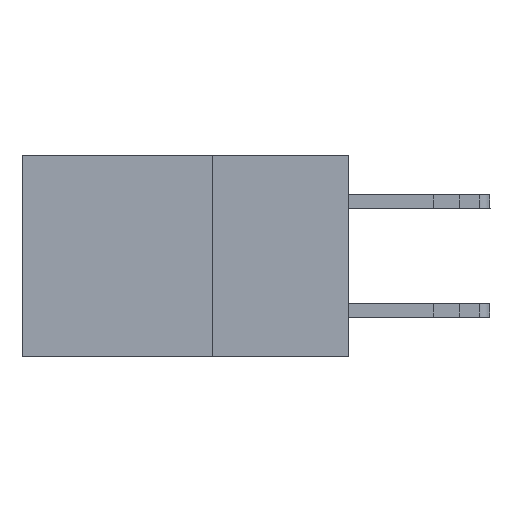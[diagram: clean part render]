
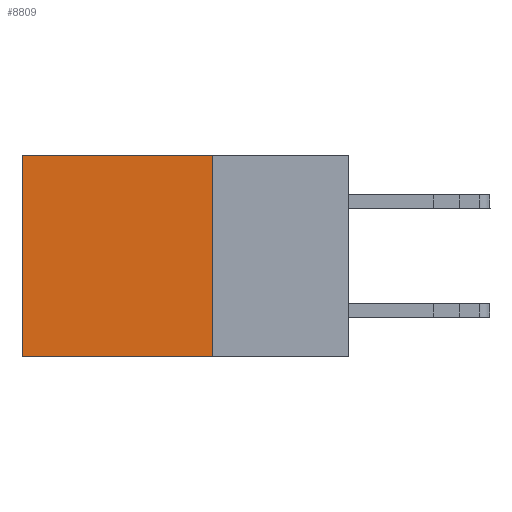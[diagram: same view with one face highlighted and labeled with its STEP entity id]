
A CAD part, left-side view. The second image highlights one B-rep face of the part: STEP entity #8809.
In plain terms, the highlighted planar face has unit normal (-1, 0, 0).
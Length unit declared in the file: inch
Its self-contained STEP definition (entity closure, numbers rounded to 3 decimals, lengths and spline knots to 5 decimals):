
#132 = EDGE_LOOP ( 'NONE', ( #5595, #189, #4515, #11271 ) ) ;
#189 = ORIENTED_EDGE ( 'NONE', *, *, #10276, .F. ) ;
#802 = DIRECTION ( 'NONE',  ( 0., 1., 0. ) ) ;
#1008 = EDGE_CURVE ( 'NONE', #4295, #7674, #4950, .T. ) ;
#1892 = VECTOR ( 'NONE', #4882, 39.37008 ) ;
#3002 = VERTEX_POINT ( 'NONE', #4215 ) ;
#3110 = VECTOR ( 'NONE', #9646, 39.37008 ) ;
#3763 = LINE ( 'NONE', #10291, #5904 ) ;
#3875 = AXIS2_PLACEMENT_3D ( 'NONE', #6365, #10100, #10986 ) ;
#3936 = LINE ( 'NONE', #6600, #3110 ) ;
#4215 = CARTESIAN_POINT ( 'NONE',  ( 0.298, 0.6, -0.37 ) ) ;
#4295 = VERTEX_POINT ( 'NONE', #5950 ) ;
#4413 = DIRECTION ( 'NONE',  ( 0., 1., 0. ) ) ;
#4515 = ORIENTED_EDGE ( 'NONE', *, *, #1008, .F. ) ;
#4850 = VECTOR ( 'NONE', #4413, 39.37008 ) ;
#4882 = DIRECTION ( 'NONE',  ( 0., 0., -1. ) ) ;
#4950 = LINE ( 'NONE', #6855, #1892 ) ;
#5394 = EDGE_CURVE ( 'NONE', #6428, #3002, #3936, .T. ) ;
#5595 = ORIENTED_EDGE ( 'NONE', *, *, #5394, .T. ) ;
#5904 = VECTOR ( 'NONE', #802, 39.37008 ) ;
#5950 = CARTESIAN_POINT ( 'NONE',  ( 0.298, 0.25, 0. ) ) ;
#6365 = CARTESIAN_POINT ( 'NONE',  ( 0.298, 0.25, 0. ) ) ;
#6428 = VERTEX_POINT ( 'NONE', #10631 ) ;
#6600 = CARTESIAN_POINT ( 'NONE',  ( 0.298, 0.6, 0. ) ) ;
#6855 = CARTESIAN_POINT ( 'NONE',  ( 0.298, 0.25, 0. ) ) ;
#7131 = FACE_OUTER_BOUND ( 'NONE', #132, .T. ) ;
#7674 = VERTEX_POINT ( 'NONE', #7678 ) ;
#7678 = CARTESIAN_POINT ( 'NONE',  ( 0.298, 0.25, -0.37 ) ) ;
#8341 = CARTESIAN_POINT ( 'NONE',  ( 0.298, 0.25, 0. ) ) ;
#8809 = ADVANCED_FACE ( 'NONE', ( #7131 ), #11177, .F. ) ;
#9646 = DIRECTION ( 'NONE',  ( 0., 0., -1. ) ) ;
#10100 = DIRECTION ( 'NONE',  ( 1., 0., 0. ) ) ;
#10276 = EDGE_CURVE ( 'NONE', #7674, #3002, #3763, .T. ) ;
#10291 = CARTESIAN_POINT ( 'NONE',  ( 0.298, 0.25, -0.37 ) ) ;
#10365 = LINE ( 'NONE', #8341, #4850 ) ;
#10631 = CARTESIAN_POINT ( 'NONE',  ( 0.298, 0.6, 0. ) ) ;
#10986 = DIRECTION ( 'NONE',  ( 0., 0., -1. ) ) ;
#11177 = PLANE ( 'NONE',  #3875 ) ;
#11271 = ORIENTED_EDGE ( 'NONE', *, *, #12015, .T. ) ;
#12015 = EDGE_CURVE ( 'NONE', #4295, #6428, #10365, .T. ) ;
